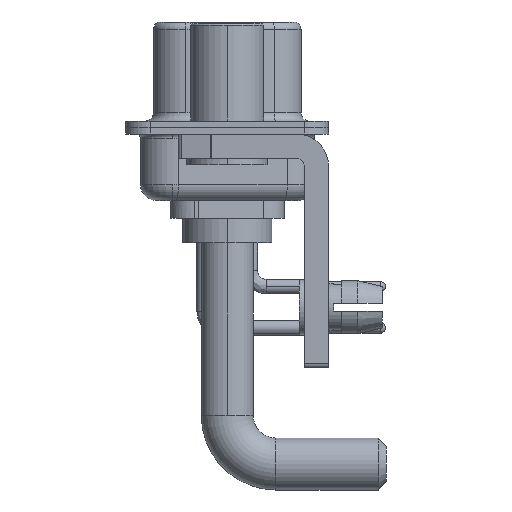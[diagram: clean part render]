
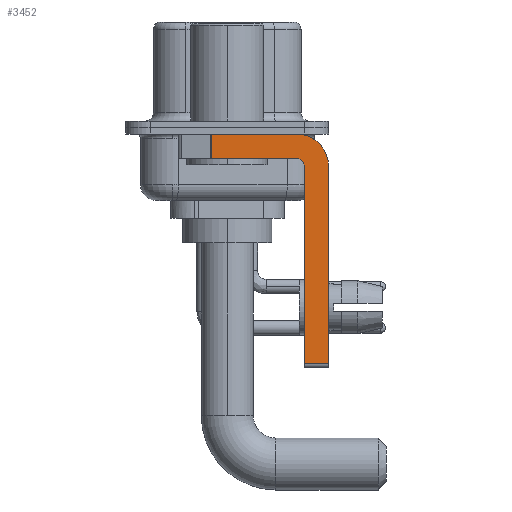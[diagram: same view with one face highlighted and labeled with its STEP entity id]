
A CAD part, left-side view. The second image highlights one B-rep face of the part: STEP entity #3452.
In plain terms, the highlighted planar face has unit normal (-1, 0, 0).
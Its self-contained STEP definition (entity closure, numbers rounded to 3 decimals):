
#134 = VERTEX_POINT ( 'NONE', #6370 ) ;
#566 = CARTESIAN_POINT ( 'NONE',  ( -2.9, -4.25, -2.4 ) ) ;
#788 = CARTESIAN_POINT ( 'NONE',  ( -2.9, -4.25, -1.9 ) ) ;
#937 = EDGE_CURVE ( 'NONE', #9369, #26359, #19725, .T. ) ;
#1326 = CARTESIAN_POINT ( 'NONE',  ( -2.9, -4.75, -2.4 ) ) ;
#1650 = CARTESIAN_POINT ( 'NONE',  ( -2.9, -4.75, -14.8 ) ) ;
#1812 = AXIS2_PLACEMENT_3D ( 'NONE', #24434, #24305, #22149 ) ;
#1922 = ORIENTED_EDGE ( 'NONE', *, *, #4763, .F. ) ;
#2702 = VERTEX_POINT ( 'NONE', #25236 ) ;
#2952 = VECTOR ( 'NONE', #18784, 1000. ) ;
#3171 = VERTEX_POINT ( 'NONE', #26258 ) ;
#3452 = ADVANCED_FACE ( 'NONE', ( #25429 ), #14948, .F. ) ;
#3592 = EDGE_CURVE ( 'NONE', #9369, #16835, #22058, .T. ) ;
#3719 = LINE ( 'NONE', #21962, #22642 ) ;
#3851 = DIRECTION ( 'NONE',  ( 0., 0., -1. ) ) ;
#3923 = AXIS2_PLACEMENT_3D ( 'NONE', #566, #7173, #11042 ) ;
#4104 = CARTESIAN_POINT ( 'NONE',  ( -2.9, -4.25, -1.9 ) ) ;
#4763 = EDGE_CURVE ( 'NONE', #16835, #5605, #25864, .T. ) ;
#4875 = ORIENTED_EDGE ( 'NONE', *, *, #11702, .F. ) ;
#5177 = ORIENTED_EDGE ( 'NONE', *, *, #937, .T. ) ;
#5605 = VERTEX_POINT ( 'NONE', #4104 ) ;
#6132 = VERTEX_POINT ( 'NONE', #24472 ) ;
#6370 = CARTESIAN_POINT ( 'NONE',  ( -2.9, 0.978, -1.9 ) ) ;
#6743 = DIRECTION ( 'NONE',  ( 0., 0., -1. ) ) ;
#7173 = DIRECTION ( 'NONE',  ( 1., 0., 0. ) ) ;
#8766 = CIRCLE ( 'NONE', #14325, 2. ) ;
#9369 = VERTEX_POINT ( 'NONE', #11893 ) ;
#9373 = ORIENTED_EDGE ( 'NONE', *, *, #26397, .F. ) ;
#9381 = ORIENTED_EDGE ( 'NONE', *, *, #18783, .F. ) ;
#10018 = VECTOR ( 'NONE', #24039, 1000. ) ;
#11042 = DIRECTION ( 'NONE',  ( 0., 0., -1. ) ) ;
#11702 = EDGE_CURVE ( 'NONE', #6132, #3171, #18145, .T. ) ;
#11854 = DIRECTION ( 'NONE',  ( 0., -1., 0. ) ) ;
#11893 = CARTESIAN_POINT ( 'NONE',  ( -2.9, -4.75, -14.55 ) ) ;
#12637 = CARTESIAN_POINT ( 'NONE',  ( -2.9, -4.25, -2.4 ) ) ;
#14325 = AXIS2_PLACEMENT_3D ( 'NONE', #12637, #17058, #6743 ) ;
#14948 = PLANE ( 'NONE',  #3923 ) ;
#16154 = EDGE_LOOP ( 'NONE', ( #4875, #23636, #22090, #1922, #16810, #5177, #9373, #9381 ) ) ;
#16437 = VECTOR ( 'NONE', #11854, 1000. ) ;
#16720 = EDGE_CURVE ( 'NONE', #5605, #134, #16908, .T. ) ;
#16810 = ORIENTED_EDGE ( 'NONE', *, *, #3592, .F. ) ;
#16835 = VERTEX_POINT ( 'NONE', #1326 ) ;
#16908 = LINE ( 'NONE', #788, #21610 ) ;
#17058 = DIRECTION ( 'NONE',  ( 1., 0., 0. ) ) ;
#17743 = DIRECTION ( 'NONE',  ( 0., 0., 1. ) ) ;
#18089 = CARTESIAN_POINT ( 'NONE',  ( -2.9, -4.25, -14.55 ) ) ;
#18145 = LINE ( 'NONE', #18549, #16437 ) ;
#18549 = CARTESIAN_POINT ( 'NONE',  ( -2.9, 3., -0.4 ) ) ;
#18783 = EDGE_CURVE ( 'NONE', #3171, #2702, #8766, .T. ) ;
#18784 = DIRECTION ( 'NONE',  ( 0., 0., -1. ) ) ;
#19175 = LINE ( 'NONE', #23219, #2952 ) ;
#19725 = LINE ( 'NONE', #18089, #10018 ) ;
#21501 = VECTOR ( 'NONE', #17743, 1000. ) ;
#21610 = VECTOR ( 'NONE', #22967, 1000. ) ;
#21962 = CARTESIAN_POINT ( 'NONE',  ( -2.9, 0.978, -1.9 ) ) ;
#22030 = CARTESIAN_POINT ( 'NONE',  ( -2.9, -6.25, -14.55 ) ) ;
#22058 = LINE ( 'NONE', #1650, #21501 ) ;
#22090 = ORIENTED_EDGE ( 'NONE', *, *, #16720, .F. ) ;
#22149 = DIRECTION ( 'NONE',  ( 0., 0., 1. ) ) ;
#22642 = VECTOR ( 'NONE', #3851, 1000. ) ;
#22967 = DIRECTION ( 'NONE',  ( 0., 1., 0. ) ) ;
#23219 = CARTESIAN_POINT ( 'NONE',  ( -2.9, -6.25, -2.4 ) ) ;
#23636 = ORIENTED_EDGE ( 'NONE', *, *, #25336, .T. ) ;
#24039 = DIRECTION ( 'NONE',  ( 0., -1., 0. ) ) ;
#24305 = DIRECTION ( 'NONE',  ( -1., 0., 0. ) ) ;
#24434 = CARTESIAN_POINT ( 'NONE',  ( -2.9, -4.25, -2.4 ) ) ;
#24472 = CARTESIAN_POINT ( 'NONE',  ( -2.9, 0.978, -0.4 ) ) ;
#25236 = CARTESIAN_POINT ( 'NONE',  ( -2.9, -6.25, -2.4 ) ) ;
#25336 = EDGE_CURVE ( 'NONE', #6132, #134, #3719, .T. ) ;
#25429 = FACE_OUTER_BOUND ( 'NONE', #16154, .T. ) ;
#25864 = CIRCLE ( 'NONE', #1812, 0.5 ) ;
#26258 = CARTESIAN_POINT ( 'NONE',  ( -2.9, -4.25, -0.4 ) ) ;
#26359 = VERTEX_POINT ( 'NONE', #22030 ) ;
#26397 = EDGE_CURVE ( 'NONE', #2702, #26359, #19175, .T. ) ;
